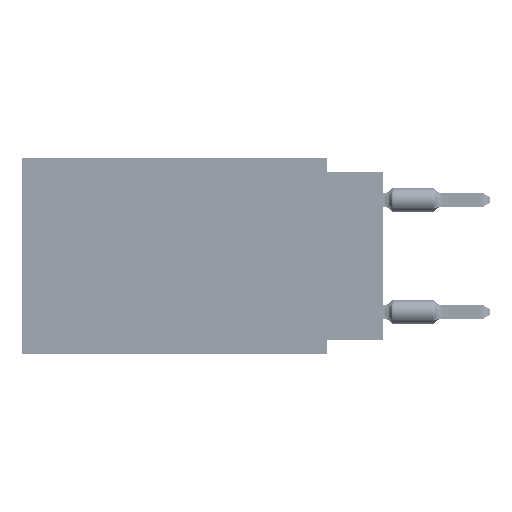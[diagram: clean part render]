
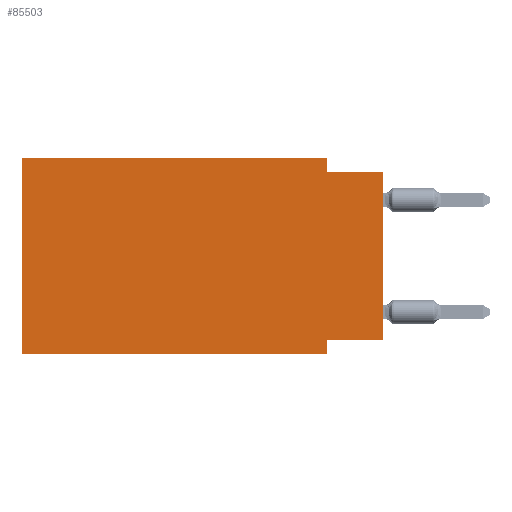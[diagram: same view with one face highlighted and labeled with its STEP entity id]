
A CAD part, left-side view. The second image highlights one B-rep face of the part: STEP entity #85503.
In plain terms, the highlighted planar face has unit normal (-1, 0, 0).
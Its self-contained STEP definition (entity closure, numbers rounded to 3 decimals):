
#3518 = VERTEX_POINT ( 'NONE', #89595 ) ;
#7671 = EDGE_CURVE ( 'NONE', #103935, #65051, #67344, .T. ) ;
#8657 = VECTOR ( 'NONE', #56316, 1000. ) ;
#8731 = CARTESIAN_POINT ( 'NONE',  ( 0., 16.383, 0. ) ) ;
#9159 = CARTESIAN_POINT ( 'NONE',  ( 0., 16.383, -8.89 ) ) ;
#9163 = VECTOR ( 'NONE', #41429, 1000. ) ;
#10231 = VERTEX_POINT ( 'NONE', #54136 ) ;
#10515 = ORIENTED_EDGE ( 'NONE', *, *, #15477, .F. ) ;
#11658 = DIRECTION ( 'NONE',  ( 0., 0., 1. ) ) ;
#11669 = DIRECTION ( 'NONE',  ( 0., -1., 0. ) ) ;
#11761 = CARTESIAN_POINT ( 'NONE',  ( 0., 0., -8.255 ) ) ;
#12615 = EDGE_CURVE ( 'NONE', #10231, #97894, #79418, .T. ) ;
#14023 = DIRECTION ( 'NONE',  ( 0., 0., -1. ) ) ;
#14538 = LINE ( 'NONE', #63254, #92320 ) ;
#14805 = DIRECTION ( 'NONE',  ( 0., 1., 0. ) ) ;
#15477 = EDGE_CURVE ( 'NONE', #103850, #52435, #92205, .T. ) ;
#17093 = FACE_OUTER_BOUND ( 'NONE', #42098, .T. ) ;
#24016 = LINE ( 'NONE', #31932, #8657 ) ;
#26591 = PLANE ( 'NONE',  #48693 ) ;
#29356 = EDGE_CURVE ( 'NONE', #10231, #52435, #68865, .T. ) ;
#31932 = CARTESIAN_POINT ( 'NONE',  ( 0., 2.54, 0. ) ) ;
#37008 = VECTOR ( 'NONE', #59402, 1000. ) ;
#37045 = CARTESIAN_POINT ( 'NONE',  ( 0., 0., 0. ) ) ;
#37635 = ORIENTED_EDGE ( 'NONE', *, *, #12615, .F. ) ;
#40970 = ORIENTED_EDGE ( 'NONE', *, *, #97743, .T. ) ;
#41429 = DIRECTION ( 'NONE',  ( 0., -1., 0. ) ) ;
#42098 = EDGE_LOOP ( 'NONE', ( #93171, #10515, #94668, #43227, #96405, #40970, #71974, #37635 ) ) ;
#42934 = CARTESIAN_POINT ( 'NONE',  ( 0., 0., -0.635 ) ) ;
#43227 = ORIENTED_EDGE ( 'NONE', *, *, #92128, .F. ) ;
#47926 = VECTOR ( 'NONE', #11669, 1000. ) ;
#48693 = AXIS2_PLACEMENT_3D ( 'NONE', #90699, #67358, #49353 ) ;
#49353 = DIRECTION ( 'NONE',  ( 0., 0., -1. ) ) ;
#49477 = DIRECTION ( 'NONE',  ( 0., -1., 0. ) ) ;
#52209 = CARTESIAN_POINT ( 'NONE',  ( 0., 2.54, -8.89 ) ) ;
#52435 = VERTEX_POINT ( 'NONE', #77814 ) ;
#54136 = CARTESIAN_POINT ( 'NONE',  ( 0., 0., -8.255 ) ) ;
#54679 = VECTOR ( 'NONE', #49477, 1000. ) ;
#56316 = DIRECTION ( 'NONE',  ( 0., 0., -1. ) ) ;
#59402 = DIRECTION ( 'NONE',  ( 0., 0., 1. ) ) ;
#59461 = EDGE_CURVE ( 'NONE', #97894, #81805, #14538, .T. ) ;
#63254 = CARTESIAN_POINT ( 'NONE',  ( 0., 2.54, -8.89 ) ) ;
#65051 = VERTEX_POINT ( 'NONE', #74911 ) ;
#67344 = LINE ( 'NONE', #99659, #37008 ) ;
#67358 = DIRECTION ( 'NONE',  ( 1., 0., 0. ) ) ;
#68865 = LINE ( 'NONE', #37045, #72410 ) ;
#71974 = ORIENTED_EDGE ( 'NONE', *, *, #59461, .F. ) ;
#72410 = VECTOR ( 'NONE', #11658, 1000. ) ;
#74911 = CARTESIAN_POINT ( 'NONE',  ( 0., 16.383, 0. ) ) ;
#77659 = LINE ( 'NONE', #8731, #54679 ) ;
#77814 = CARTESIAN_POINT ( 'NONE',  ( 0., 0., -0.635 ) ) ;
#79418 = LINE ( 'NONE', #11761, #98235 ) ;
#81737 = LINE ( 'NONE', #9159, #9163 ) ;
#81805 = VERTEX_POINT ( 'NONE', #52209 ) ;
#85503 = ADVANCED_FACE ( 'NONE', ( #17093 ), #26591, .F. ) ;
#85975 = CARTESIAN_POINT ( 'NONE',  ( 0., 2.54, -0.635 ) ) ;
#87929 = EDGE_CURVE ( 'NONE', #3518, #103850, #24016, .T. ) ;
#89595 = CARTESIAN_POINT ( 'NONE',  ( 0., 2.54, 0. ) ) ;
#90699 = CARTESIAN_POINT ( 'NONE',  ( 0., 16.383, 0. ) ) ;
#92128 = EDGE_CURVE ( 'NONE', #65051, #3518, #77659, .T. ) ;
#92205 = LINE ( 'NONE', #42934, #47926 ) ;
#92320 = VECTOR ( 'NONE', #14023, 1000. ) ;
#93171 = ORIENTED_EDGE ( 'NONE', *, *, #29356, .T. ) ;
#94444 = CARTESIAN_POINT ( 'NONE',  ( 0., 16.383, -8.89 ) ) ;
#94668 = ORIENTED_EDGE ( 'NONE', *, *, #87929, .F. ) ;
#96405 = ORIENTED_EDGE ( 'NONE', *, *, #7671, .F. ) ;
#97743 = EDGE_CURVE ( 'NONE', #103935, #81805, #81737, .T. ) ;
#97894 = VERTEX_POINT ( 'NONE', #100734 ) ;
#98235 = VECTOR ( 'NONE', #14805, 1000. ) ;
#99659 = CARTESIAN_POINT ( 'NONE',  ( 0., 16.383, 0. ) ) ;
#100734 = CARTESIAN_POINT ( 'NONE',  ( 0., 2.54, -8.255 ) ) ;
#103850 = VERTEX_POINT ( 'NONE', #85975 ) ;
#103935 = VERTEX_POINT ( 'NONE', #94444 ) ;
